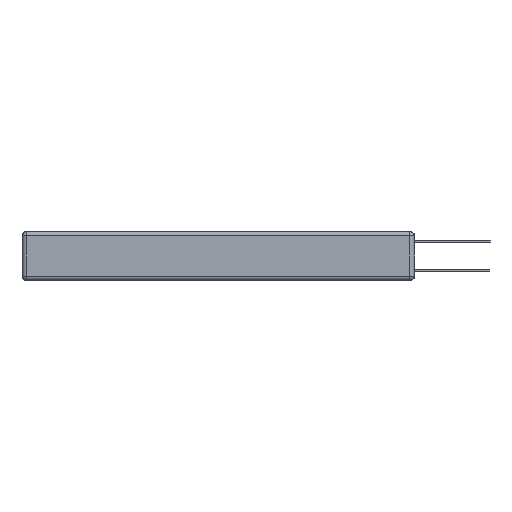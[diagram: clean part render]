
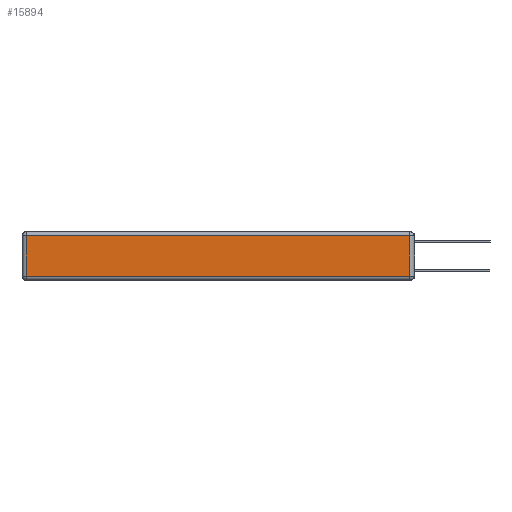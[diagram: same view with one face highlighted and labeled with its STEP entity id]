
A CAD part, left-side view. The second image highlights one B-rep face of the part: STEP entity #15894.
In plain terms, the highlighted planar face has unit normal (-1, 0, 0).
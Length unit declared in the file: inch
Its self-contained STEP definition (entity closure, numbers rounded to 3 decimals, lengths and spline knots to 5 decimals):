
#1931 = DIRECTION ( 'NONE',  ( -1., 0., 0. ) ) ;
#2210 = LINE ( 'NONE', #21138, #22255 ) ;
#2847 = CARTESIAN_POINT ( 'NONE',  ( 0., 2.72, -0.343 ) ) ;
#3507 = CARTESIAN_POINT ( 'NONE',  ( 0., 0.03, -0.03 ) ) ;
#3659 = VERTEX_POINT ( 'NONE', #3507 ) ;
#4637 = LINE ( 'NONE', #10445, #9378 ) ;
#5117 = CARTESIAN_POINT ( 'NONE',  ( 0., 2.72, -0.03 ) ) ;
#5972 = VERTEX_POINT ( 'NONE', #19987 ) ;
#6098 = EDGE_CURVE ( 'NONE', #8273, #5972, #4637, .T. ) ;
#7116 = DIRECTION ( 'NONE',  ( 0., 1., 0. ) ) ;
#7806 = ORIENTED_EDGE ( 'NONE', *, *, #6098, .T. ) ;
#7945 = CARTESIAN_POINT ( 'NONE',  ( 0., 0., -0.343 ) ) ;
#8273 = VERTEX_POINT ( 'NONE', #8932 ) ;
#8932 = CARTESIAN_POINT ( 'NONE',  ( 0., 2.72, -0.313 ) ) ;
#9346 = DIRECTION ( 'NONE',  ( 0., 0., 1. ) ) ;
#9378 = VECTOR ( 'NONE', #12478, 39.37008 ) ;
#10445 = CARTESIAN_POINT ( 'NONE',  ( 0., 0., -0.313 ) ) ;
#10639 = VERTEX_POINT ( 'NONE', #5117 ) ;
#11218 = FACE_OUTER_BOUND ( 'NONE', #21762, .T. ) ;
#12383 = ORIENTED_EDGE ( 'NONE', *, *, #20819, .T. ) ;
#12478 = DIRECTION ( 'NONE',  ( 0., -1., 0. ) ) ;
#13026 = EDGE_CURVE ( 'NONE', #5972, #3659, #19237, .T. ) ;
#13474 = VECTOR ( 'NONE', #16906, 39.37008 ) ;
#14024 = PLANE ( 'NONE',  #19396 ) ;
#15894 = ADVANCED_FACE ( 'NONE', ( #11218 ), #14024, .T. ) ;
#16017 = DIRECTION ( 'NONE',  ( 0., 0., 1. ) ) ;
#16906 = DIRECTION ( 'NONE',  ( 0., 0., -1. ) ) ;
#18127 = LINE ( 'NONE', #2847, #13474 ) ;
#19237 = LINE ( 'NONE', #21238, #23877 ) ;
#19396 = AXIS2_PLACEMENT_3D ( 'NONE', #7945, #1931, #16017 ) ;
#19827 = ORIENTED_EDGE ( 'NONE', *, *, #23163, .T. ) ;
#19987 = CARTESIAN_POINT ( 'NONE',  ( 0., 0.03, -0.313 ) ) ;
#20819 = EDGE_CURVE ( 'NONE', #3659, #10639, #2210, .T. ) ;
#21138 = CARTESIAN_POINT ( 'NONE',  ( 0., 2.75, -0.03 ) ) ;
#21238 = CARTESIAN_POINT ( 'NONE',  ( 0., 0.03, -0.343 ) ) ;
#21762 = EDGE_LOOP ( 'NONE', ( #7806, #25883, #12383, #19827 ) ) ;
#22255 = VECTOR ( 'NONE', #7116, 39.37008 ) ;
#23163 = EDGE_CURVE ( 'NONE', #10639, #8273, #18127, .T. ) ;
#23877 = VECTOR ( 'NONE', #9346, 39.37008 ) ;
#25883 = ORIENTED_EDGE ( 'NONE', *, *, #13026, .T. ) ;
